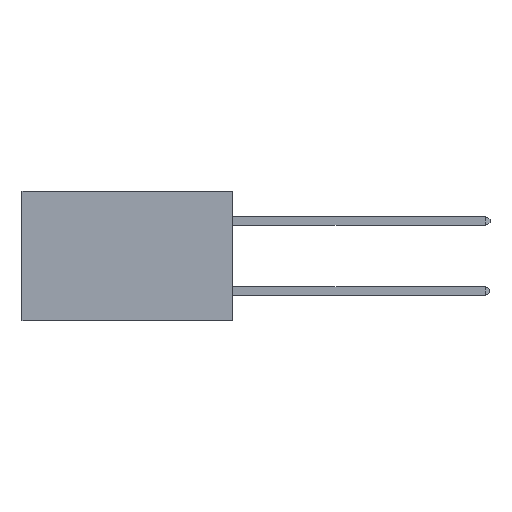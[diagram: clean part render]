
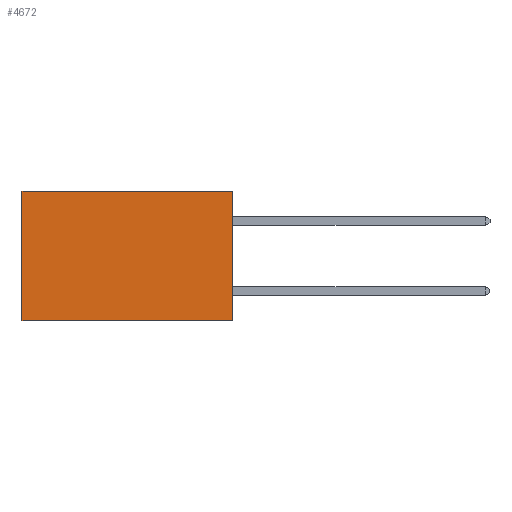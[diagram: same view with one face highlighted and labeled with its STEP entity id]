
A CAD part, left-side view. The second image highlights one B-rep face of the part: STEP entity #4672.
In plain terms, the highlighted planar face has unit normal (-1, 0, 0).
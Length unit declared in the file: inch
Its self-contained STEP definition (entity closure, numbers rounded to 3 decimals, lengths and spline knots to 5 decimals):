
#848 = DIRECTION ( 'NONE',  ( 0., 0., -1. ) ) ;
#991 = VERTEX_POINT ( 'NONE', #6093 ) ;
#1377 = DIRECTION ( 'NONE',  ( 0., 1., 0. ) ) ;
#1554 = PLANE ( 'NONE',  #6468 ) ;
#1586 = EDGE_LOOP ( 'NONE', ( #15826, #3663, #16433, #18421 ) ) ;
#1826 = FACE_OUTER_BOUND ( 'NONE', #1586, .T. ) ;
#2068 = DIRECTION ( 'NONE',  ( 0., 1., 0. ) ) ;
#3201 = LINE ( 'NONE', #20734, #16274 ) ;
#3514 = EDGE_CURVE ( 'NONE', #7651, #991, #20182, .T. ) ;
#3663 = ORIENTED_EDGE ( 'NONE', *, *, #20448, .F. ) ;
#4164 = LINE ( 'NONE', #15002, #7615 ) ;
#4369 = CARTESIAN_POINT ( 'NONE',  ( 0.2875, 0.6, 0. ) ) ;
#4672 = ADVANCED_FACE ( 'NONE', ( #1826 ), #1554, .F. ) ;
#6093 = CARTESIAN_POINT ( 'NONE',  ( 0.2875, 0.6, -0.37 ) ) ;
#6468 = AXIS2_PLACEMENT_3D ( 'NONE', #18583, #8397, #20230 ) ;
#7176 = EDGE_CURVE ( 'NONE', #18384, #7651, #4164, .T. ) ;
#7615 = VECTOR ( 'NONE', #1377, 39.37008 ) ;
#7651 = VERTEX_POINT ( 'NONE', #4369 ) ;
#7714 = CARTESIAN_POINT ( 'NONE',  ( 0.2875, 0.6, 0. ) ) ;
#8397 = DIRECTION ( 'NONE',  ( 1., 0., 0. ) ) ;
#10713 = EDGE_CURVE ( 'NONE', #18384, #16652, #17127, .T. ) ;
#15002 = CARTESIAN_POINT ( 'NONE',  ( 0.2875, 0., 0. ) ) ;
#15766 = VECTOR ( 'NONE', #848, 39.37008 ) ;
#15826 = ORIENTED_EDGE ( 'NONE', *, *, #3514, .T. ) ;
#16098 = DIRECTION ( 'NONE',  ( 0., 0., -1. ) ) ;
#16274 = VECTOR ( 'NONE', #2068, 39.37008 ) ;
#16433 = ORIENTED_EDGE ( 'NONE', *, *, #10713, .F. ) ;
#16652 = VERTEX_POINT ( 'NONE', #18735 ) ;
#17127 = LINE ( 'NONE', #21105, #21528 ) ;
#18384 = VERTEX_POINT ( 'NONE', #21814 ) ;
#18421 = ORIENTED_EDGE ( 'NONE', *, *, #7176, .T. ) ;
#18583 = CARTESIAN_POINT ( 'NONE',  ( 0.2875, 0., 0. ) ) ;
#18735 = CARTESIAN_POINT ( 'NONE',  ( 0.2875, 0., -0.37 ) ) ;
#20182 = LINE ( 'NONE', #7714, #15766 ) ;
#20230 = DIRECTION ( 'NONE',  ( 0., 0., -1. ) ) ;
#20448 = EDGE_CURVE ( 'NONE', #16652, #991, #3201, .T. ) ;
#20734 = CARTESIAN_POINT ( 'NONE',  ( 0.2875, 0., -0.37 ) ) ;
#21105 = CARTESIAN_POINT ( 'NONE',  ( 0.2875, 0., 0. ) ) ;
#21528 = VECTOR ( 'NONE', #16098, 39.37008 ) ;
#21814 = CARTESIAN_POINT ( 'NONE',  ( 0.2875, 0., 0. ) ) ;
